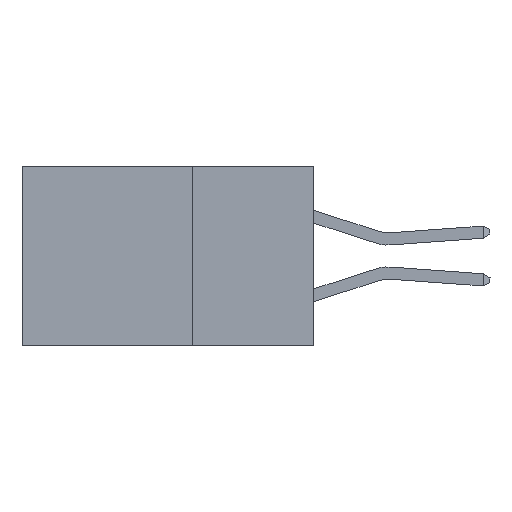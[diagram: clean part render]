
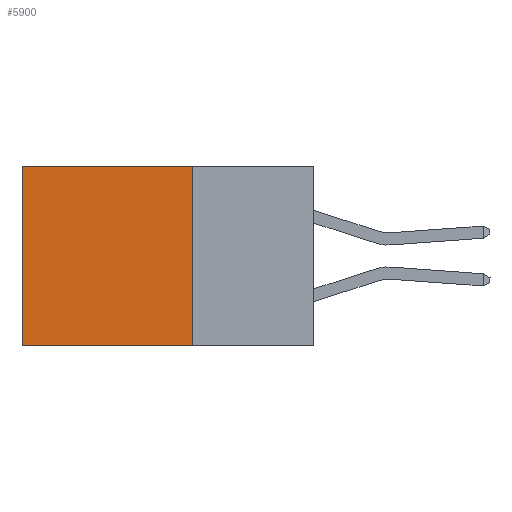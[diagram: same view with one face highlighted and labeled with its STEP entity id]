
A CAD part, left-side view. The second image highlights one B-rep face of the part: STEP entity #5900.
In plain terms, the highlighted planar face has unit normal (-1, 0, 0).
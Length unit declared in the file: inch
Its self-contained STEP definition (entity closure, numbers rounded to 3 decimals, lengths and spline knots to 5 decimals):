
#48 = CARTESIAN_POINT ( 'NONE',  ( 0.2875, 0.6, -0.37 ) ) ;
#959 = CARTESIAN_POINT ( 'NONE',  ( 0.2875, 0.25, 0. ) ) ;
#1210 = DIRECTION ( 'NONE',  ( 0., 0., -1. ) ) ;
#2509 = VERTEX_POINT ( 'NONE', #8330 ) ;
#3952 = ORIENTED_EDGE ( 'NONE', *, *, #14688, .F. ) ;
#4130 = VECTOR ( 'NONE', #12389, 39.37008 ) ;
#4650 = VERTEX_POINT ( 'NONE', #10373 ) ;
#4732 = DIRECTION ( 'NONE',  ( 0., 0., -1. ) ) ;
#4762 = DIRECTION ( 'NONE',  ( 0., 1., 0. ) ) ;
#4787 = EDGE_LOOP ( 'NONE', ( #12091, #11609, #3952, #5446 ) ) ;
#5064 = VECTOR ( 'NONE', #4732, 39.37008 ) ;
#5446 = ORIENTED_EDGE ( 'NONE', *, *, #15070, .T. ) ;
#5612 = AXIS2_PLACEMENT_3D ( 'NONE', #10743, #17181, #1210 ) ;
#5900 = ADVANCED_FACE ( 'NONE', ( #11754 ), #6746, .F. ) ;
#6746 = PLANE ( 'NONE',  #5612 ) ;
#7904 = LINE ( 'NONE', #17642, #15106 ) ;
#8330 = CARTESIAN_POINT ( 'NONE',  ( 0.2875, 0.25, 0. ) ) ;
#8585 = VECTOR ( 'NONE', #14453, 39.37008 ) ;
#9218 = LINE ( 'NONE', #959, #4130 ) ;
#9237 = LINE ( 'NONE', #16168, #8585 ) ;
#10373 = CARTESIAN_POINT ( 'NONE',  ( 0.2875, 0.6, 0. ) ) ;
#10743 = CARTESIAN_POINT ( 'NONE',  ( 0.2875, 0.25, 0. ) ) ;
#11609 = ORIENTED_EDGE ( 'NONE', *, *, #14074, .F. ) ;
#11754 = FACE_OUTER_BOUND ( 'NONE', #4787, .T. ) ;
#12091 = ORIENTED_EDGE ( 'NONE', *, *, #13390, .T. ) ;
#12181 = VERTEX_POINT ( 'NONE', #48 ) ;
#12389 = DIRECTION ( 'NONE',  ( 0., 0., -1. ) ) ;
#13390 = EDGE_CURVE ( 'NONE', #4650, #12181, #17003, .T. ) ;
#13559 = CARTESIAN_POINT ( 'NONE',  ( 0.2875, 0.25, -0.37 ) ) ;
#14074 = EDGE_CURVE ( 'NONE', #18017, #12181, #9237, .T. ) ;
#14453 = DIRECTION ( 'NONE',  ( 0., 1., 0. ) ) ;
#14688 = EDGE_CURVE ( 'NONE', #2509, #18017, #9218, .T. ) ;
#14834 = CARTESIAN_POINT ( 'NONE',  ( 0.2875, 0.6, 0. ) ) ;
#15070 = EDGE_CURVE ( 'NONE', #2509, #4650, #7904, .T. ) ;
#15106 = VECTOR ( 'NONE', #4762, 39.37008 ) ;
#16168 = CARTESIAN_POINT ( 'NONE',  ( 0.2875, 0.25, -0.37 ) ) ;
#17003 = LINE ( 'NONE', #14834, #5064 ) ;
#17181 = DIRECTION ( 'NONE',  ( 1., 0., 0. ) ) ;
#17642 = CARTESIAN_POINT ( 'NONE',  ( 0.2875, 0.25, 0. ) ) ;
#18017 = VERTEX_POINT ( 'NONE', #13559 ) ;
